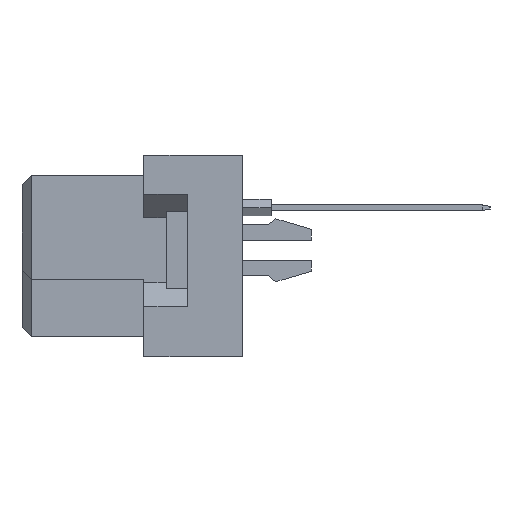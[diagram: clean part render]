
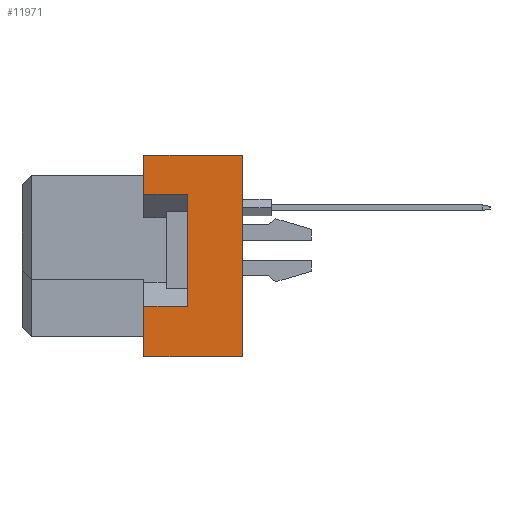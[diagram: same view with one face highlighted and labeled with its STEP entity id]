
A CAD part, left-side view. The second image highlights one B-rep face of the part: STEP entity #11971.
In plain terms, the highlighted planar face has unit normal (-1, 0, 0).
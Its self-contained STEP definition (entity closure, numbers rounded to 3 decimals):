
#45 = LINE ( 'NONE', #11740, #20264 ) ;
#80 = VERTEX_POINT ( 'NONE', #16013 ) ;
#370 = EDGE_LOOP ( 'NONE', ( #13013, #11139, #25338, #24043, #24298, #31283, #34970, #19990 ) ) ;
#754 = CARTESIAN_POINT ( 'NONE',  ( -47.5, -8.7, -2.65 ) ) ;
#1015 = EDGE_CURVE ( 'NONE', #29196, #80, #22978, .T. ) ;
#2032 = CARTESIAN_POINT ( 'NONE',  ( -47.5, -11.6, -5.3 ) ) ;
#2262 = EDGE_CURVE ( 'NONE', #13752, #80, #31738, .T. ) ;
#3197 = CARTESIAN_POINT ( 'NONE',  ( -47.5, -6.4, -5.3 ) ) ;
#3480 = CARTESIAN_POINT ( 'NONE',  ( -47.5, -11.6, -5.3 ) ) ;
#3559 = LINE ( 'NONE', #19188, #25870 ) ;
#4910 = FACE_OUTER_BOUND ( 'NONE', #370, .T. ) ;
#5025 = DIRECTION ( 'NONE',  ( 0., 1., 0. ) ) ;
#5414 = VECTOR ( 'NONE', #19865, 1000. ) ;
#5554 = EDGE_CURVE ( 'NONE', #29844, #17592, #3559, .T. ) ;
#7686 = CARTESIAN_POINT ( 'NONE',  ( -47.5, -11.6, 5.3 ) ) ;
#7996 = LINE ( 'NONE', #29154, #5414 ) ;
#8883 = VERTEX_POINT ( 'NONE', #9614 ) ;
#9089 = DIRECTION ( 'NONE',  ( 0., 0., 1. ) ) ;
#9614 = CARTESIAN_POINT ( 'NONE',  ( -47.5, -6.4, -5.3 ) ) ;
#11139 = ORIENTED_EDGE ( 'NONE', *, *, #24723, .F. ) ;
#11204 = VECTOR ( 'NONE', #23003, 1000. ) ;
#11740 = CARTESIAN_POINT ( 'NONE',  ( -47.5, -8.7, -2.65 ) ) ;
#11915 = DIRECTION ( 'NONE',  ( 0., 0., 1. ) ) ;
#11971 = ADVANCED_FACE ( 'NONE', ( #4910 ), #19552, .T. ) ;
#13013 = ORIENTED_EDGE ( 'NONE', *, *, #5554, .T. ) ;
#13752 = VERTEX_POINT ( 'NONE', #37952 ) ;
#14293 = LINE ( 'NONE', #2032, #11204 ) ;
#14448 = CARTESIAN_POINT ( 'NONE',  ( -47.5, -11.6, 5.3 ) ) ;
#15312 = CARTESIAN_POINT ( 'NONE',  ( -47.5, -8.7, 3.25 ) ) ;
#16013 = CARTESIAN_POINT ( 'NONE',  ( -47.5, -6.4, 5.3 ) ) ;
#17592 = VERTEX_POINT ( 'NONE', #18759 ) ;
#18046 = DIRECTION ( 'NONE',  ( 0., 0., 1. ) ) ;
#18759 = CARTESIAN_POINT ( 'NONE',  ( -47.5, -6.4, -2.65 ) ) ;
#19188 = CARTESIAN_POINT ( 'NONE',  ( -47.5, -8.7, -2.65 ) ) ;
#19552 = PLANE ( 'NONE',  #31657 ) ;
#19621 = DIRECTION ( 'NONE',  ( 0., 0., 1. ) ) ;
#19865 = DIRECTION ( 'NONE',  ( 0., 1., 0. ) ) ;
#19990 = ORIENTED_EDGE ( 'NONE', *, *, #25051, .F. ) ;
#20055 = CARTESIAN_POINT ( 'NONE',  ( -47.5, -11.6, 5.3 ) ) ;
#20264 = VECTOR ( 'NONE', #18046, 1000. ) ;
#21285 = EDGE_CURVE ( 'NONE', #30177, #13752, #36172, .T. ) ;
#21498 = VECTOR ( 'NONE', #11915, 1000. ) ;
#21861 = VECTOR ( 'NONE', #5025, 1000. ) ;
#22978 = LINE ( 'NONE', #32271, #36854 ) ;
#23003 = DIRECTION ( 'NONE',  ( 0., 1., 0. ) ) ;
#24043 = ORIENTED_EDGE ( 'NONE', *, *, #21285, .T. ) ;
#24298 = ORIENTED_EDGE ( 'NONE', *, *, #2262, .T. ) ;
#24723 = EDGE_CURVE ( 'NONE', #8883, #17592, #32684, .T. ) ;
#25051 = EDGE_CURVE ( 'NONE', #29844, #36543, #45, .T. ) ;
#25338 = ORIENTED_EDGE ( 'NONE', *, *, #36825, .F. ) ;
#25487 = DIRECTION ( 'NONE',  ( 0., 0., 1. ) ) ;
#25870 = VECTOR ( 'NONE', #36975, 1000. ) ;
#28557 = VECTOR ( 'NONE', #9089, 1000. ) ;
#29154 = CARTESIAN_POINT ( 'NONE',  ( -47.5, -8.7, 3.25 ) ) ;
#29196 = VERTEX_POINT ( 'NONE', #38062 ) ;
#29844 = VERTEX_POINT ( 'NONE', #754 ) ;
#30177 = VERTEX_POINT ( 'NONE', #3480 ) ;
#31283 = ORIENTED_EDGE ( 'NONE', *, *, #1015, .F. ) ;
#31621 = DIRECTION ( 'NONE',  ( -1., 0., 0. ) ) ;
#31657 = AXIS2_PLACEMENT_3D ( 'NONE', #7686, #31621, #25487 ) ;
#31738 = LINE ( 'NONE', #20055, #21861 ) ;
#32271 = CARTESIAN_POINT ( 'NONE',  ( -47.5, -6.4, -5.3 ) ) ;
#32684 = LINE ( 'NONE', #3197, #21498 ) ;
#34326 = EDGE_CURVE ( 'NONE', #36543, #29196, #7996, .T. ) ;
#34970 = ORIENTED_EDGE ( 'NONE', *, *, #34326, .F. ) ;
#36172 = LINE ( 'NONE', #14448, #28557 ) ;
#36543 = VERTEX_POINT ( 'NONE', #15312 ) ;
#36825 = EDGE_CURVE ( 'NONE', #30177, #8883, #14293, .T. ) ;
#36854 = VECTOR ( 'NONE', #19621, 1000. ) ;
#36975 = DIRECTION ( 'NONE',  ( 0., 1., 0. ) ) ;
#37952 = CARTESIAN_POINT ( 'NONE',  ( -47.5, -11.6, 5.3 ) ) ;
#38062 = CARTESIAN_POINT ( 'NONE',  ( -47.5, -6.4, 3.25 ) ) ;
